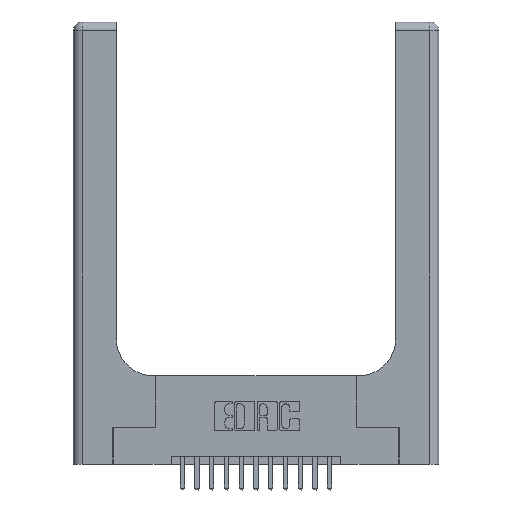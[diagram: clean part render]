
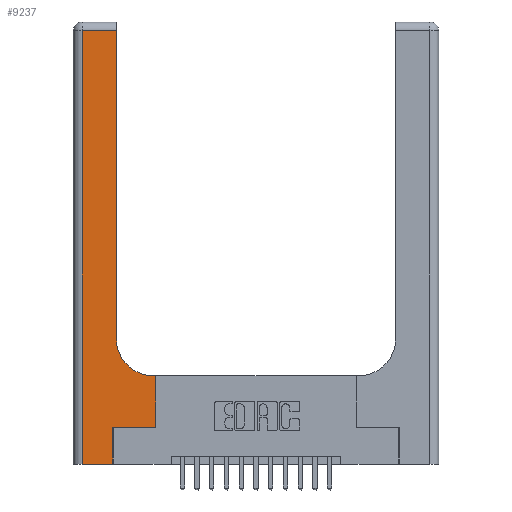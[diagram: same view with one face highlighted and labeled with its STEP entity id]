
A CAD part, top view. The second image highlights one B-rep face of the part: STEP entity #9237.
In plain terms, the highlighted planar face has unit normal (0, 0, 1).
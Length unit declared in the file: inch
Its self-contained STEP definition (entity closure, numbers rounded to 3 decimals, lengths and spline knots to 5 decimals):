
#5 = VECTOR ( 'NONE', #4733, 39.37008 ) ;
#11 = CARTESIAN_POINT ( 'NONE',  ( 0.269, 0., 0.37 ) ) ;
#115 = CIRCLE ( 'NONE', #14361, 0.25 ) ;
#826 = CARTESIAN_POINT ( 'NONE',  ( 0., 0., 0.37 ) ) ;
#1623 = VERTEX_POINT ( 'NONE', #7008 ) ;
#2029 = VERTEX_POINT ( 'NONE', #3585 ) ;
#2526 = LINE ( 'NONE', #14161, #9612 ) ;
#2703 = FACE_OUTER_BOUND ( 'NONE', #5483, .T. ) ;
#3246 = CARTESIAN_POINT ( 'NONE',  ( 0.2915, 3., 0.37 ) ) ;
#3399 = CARTESIAN_POINT ( 'NONE',  ( 0.06, 2.94, 0.37 ) ) ;
#3568 = VERTEX_POINT ( 'NONE', #16573 ) ;
#3585 = CARTESIAN_POINT ( 'NONE',  ( 0.5585, 0.6, 0.37 ) ) ;
#3635 = VERTEX_POINT ( 'NONE', #16166 ) ;
#3812 = DIRECTION ( 'NONE',  ( 1., 0., 0. ) ) ;
#4090 = CARTESIAN_POINT ( 'NONE',  ( 0.5415, 0.6, 0.37 ) ) ;
#4437 = LINE ( 'NONE', #3246, #5 ) ;
#4504 = DIRECTION ( 'NONE',  ( 0., 1., 0. ) ) ;
#4532 = ORIENTED_EDGE ( 'NONE', *, *, #10861, .T. ) ;
#4733 = DIRECTION ( 'NONE',  ( 0., 1., 0. ) ) ;
#4834 = AXIS2_PLACEMENT_3D ( 'NONE', #14763, #6519, #16103 ) ;
#5082 = ORIENTED_EDGE ( 'NONE', *, *, #15364, .T. ) ;
#5483 = EDGE_LOOP ( 'NONE', ( #10258, #13855, #10138, #4532, #5082, #15472, #9897, #12340, #7015 ) ) ;
#5598 = VERTEX_POINT ( 'NONE', #7931 ) ;
#5698 = DIRECTION ( 'NONE',  ( 0., -1., 0. ) ) ;
#5752 = CARTESIAN_POINT ( 'NONE',  ( 0.269, 0.25, 0.37 ) ) ;
#5887 = EDGE_CURVE ( 'NONE', #3635, #6446, #17983, .T. ) ;
#6446 = VERTEX_POINT ( 'NONE', #11062 ) ;
#6519 = DIRECTION ( 'NONE',  ( 0., 0., -1. ) ) ;
#6880 = VERTEX_POINT ( 'NONE', #14877 ) ;
#6999 = VERTEX_POINT ( 'NONE', #4090 ) ;
#7008 = CARTESIAN_POINT ( 'NONE',  ( 0.2915, 2.94, 0.37 ) ) ;
#7015 = ORIENTED_EDGE ( 'NONE', *, *, #10150, .T. ) ;
#7017 = DIRECTION ( 'NONE',  ( 0., 0., -1. ) ) ;
#7083 = DIRECTION ( 'NONE',  ( -1., 0., 0. ) ) ;
#7329 = VECTOR ( 'NONE', #4504, 39.37008 ) ;
#7754 = LINE ( 'NONE', #11, #7329 ) ;
#7931 = CARTESIAN_POINT ( 'NONE',  ( 0.2915, 0.85, 0.37 ) ) ;
#8105 = DIRECTION ( 'NONE',  ( -1., 0., 0. ) ) ;
#8309 = EDGE_CURVE ( 'NONE', #2029, #6999, #9356, .T. ) ;
#8458 = VECTOR ( 'NONE', #8105, 39.37008 ) ;
#9237 = ADVANCED_FACE ( 'NONE', ( #2703 ), #17399, .F. ) ;
#9315 = EDGE_CURVE ( 'NONE', #1623, #13827, #12652, .T. ) ;
#9356 = LINE ( 'NONE', #17993, #13118 ) ;
#9494 = CARTESIAN_POINT ( 'NONE',  ( 0., 2.94, 0.37 ) ) ;
#9612 = VECTOR ( 'NONE', #9994, 39.37008 ) ;
#9897 = ORIENTED_EDGE ( 'NONE', *, *, #10632, .T. ) ;
#9994 = DIRECTION ( 'NONE',  ( 0., 1., 0. ) ) ;
#10078 = VECTOR ( 'NONE', #3812, 39.37008 ) ;
#10138 = ORIENTED_EDGE ( 'NONE', *, *, #15198, .T. ) ;
#10150 = EDGE_CURVE ( 'NONE', #6999, #5598, #115, .T. ) ;
#10258 = ORIENTED_EDGE ( 'NONE', *, *, #16248, .T. ) ;
#10632 = EDGE_CURVE ( 'NONE', #6446, #2029, #2526, .T. ) ;
#10861 = EDGE_CURVE ( 'NONE', #3568, #6880, #14788, .T. ) ;
#11062 = CARTESIAN_POINT ( 'NONE',  ( 0.5585, 0.25, 0.37 ) ) ;
#12340 = ORIENTED_EDGE ( 'NONE', *, *, #8309, .T. ) ;
#12652 = LINE ( 'NONE', #9494, #8458 ) ;
#13118 = VECTOR ( 'NONE', #7083, 39.37008 ) ;
#13631 = VECTOR ( 'NONE', #5698, 39.37008 ) ;
#13827 = VERTEX_POINT ( 'NONE', #3399 ) ;
#13855 = ORIENTED_EDGE ( 'NONE', *, *, #9315, .T. ) ;
#14035 = DIRECTION ( 'NONE',  ( 1., 0., 0. ) ) ;
#14161 = CARTESIAN_POINT ( 'NONE',  ( 0.5585, 0.25, 0.37 ) ) ;
#14361 = AXIS2_PLACEMENT_3D ( 'NONE', #15262, #7017, #16587 ) ;
#14452 = VECTOR ( 'NONE', #14035, 39.37008 ) ;
#14763 = CARTESIAN_POINT ( 'NONE',  ( 0., 3., 0.37 ) ) ;
#14788 = LINE ( 'NONE', #826, #10078 ) ;
#14877 = CARTESIAN_POINT ( 'NONE',  ( 0.269, 0., 0.37 ) ) ;
#15198 = EDGE_CURVE ( 'NONE', #13827, #3568, #17610, .T. ) ;
#15262 = CARTESIAN_POINT ( 'NONE',  ( 0.5415, 0.85, 0.37 ) ) ;
#15364 = EDGE_CURVE ( 'NONE', #6880, #3635, #7754, .T. ) ;
#15472 = ORIENTED_EDGE ( 'NONE', *, *, #5887, .T. ) ;
#16103 = DIRECTION ( 'NONE',  ( -1., 0., 0. ) ) ;
#16166 = CARTESIAN_POINT ( 'NONE',  ( 0.269, 0.25, 0.37 ) ) ;
#16248 = EDGE_CURVE ( 'NONE', #5598, #1623, #4437, .T. ) ;
#16542 = CARTESIAN_POINT ( 'NONE',  ( 0.06, 3., 0.37 ) ) ;
#16573 = CARTESIAN_POINT ( 'NONE',  ( 0.06, 0., 0.37 ) ) ;
#16587 = DIRECTION ( 'NONE',  ( 1., 0., 0. ) ) ;
#17399 = PLANE ( 'NONE',  #4834 ) ;
#17610 = LINE ( 'NONE', #16542, #13631 ) ;
#17983 = LINE ( 'NONE', #5752, #14452 ) ;
#17993 = CARTESIAN_POINT ( 'NONE',  ( 0.2915, 0.6, 0.37 ) ) ;
